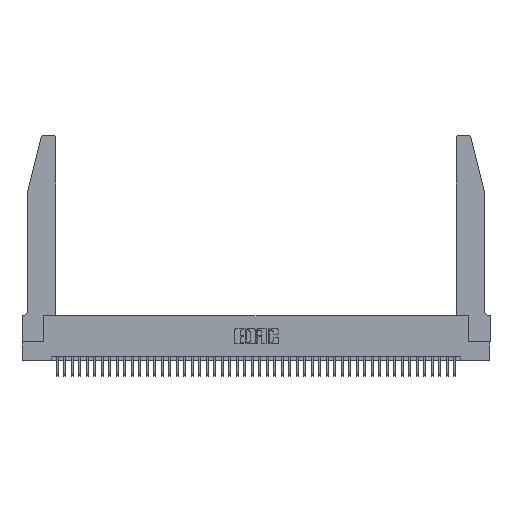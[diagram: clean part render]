
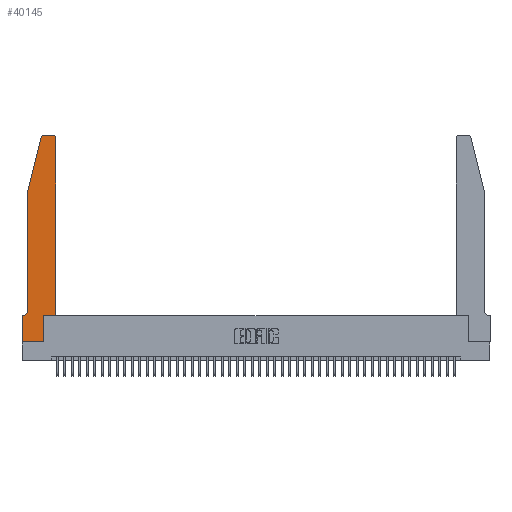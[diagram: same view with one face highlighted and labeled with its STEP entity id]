
A CAD part, top view. The second image highlights one B-rep face of the part: STEP entity #40145.
In plain terms, the highlighted planar face has unit normal (0, 0, 1).
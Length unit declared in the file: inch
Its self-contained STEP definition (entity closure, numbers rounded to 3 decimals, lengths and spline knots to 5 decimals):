
#1149 = CARTESIAN_POINT ( 'NONE',  ( 0., 0.35, 0.37 ) ) ;
#2690 = EDGE_CURVE ( 'NONE', #42190, #14684, #43488, .T. ) ;
#4485 = CIRCLE ( 'NONE', #15224, 0.03 ) ;
#4643 = EDGE_CURVE ( 'NONE', #12911, #24171, #44346, .T. ) ;
#5309 = CARTESIAN_POINT ( 'NONE',  ( 0.4505, 2.72, 0.37 ) ) ;
#5508 = ORIENTED_EDGE ( 'NONE', *, *, #18669, .T. ) ;
#6782 = CARTESIAN_POINT ( 'NONE',  ( 0., 0., 0.37 ) ) ;
#6823 = CARTESIAN_POINT ( 'NONE',  ( 0.284, 2.72, 0.37 ) ) ;
#7872 = DIRECTION ( 'NONE',  ( -0.239, -0.971, 0. ) ) ;
#8653 = DIRECTION ( 'NONE',  ( 0., 0., 1. ) ) ;
#9303 = ORIENTED_EDGE ( 'NONE', *, *, #38729, .T. ) ;
#9536 = DIRECTION ( 'NONE',  ( 0., 1., 0. ) ) ;
#9613 = CARTESIAN_POINT ( 'NONE',  ( 0.0755, 0.35, 0.37 ) ) ;
#9646 = LINE ( 'NONE', #9613, #37613 ) ;
#10460 = DIRECTION ( 'NONE',  ( 0., -1., 0. ) ) ;
#10482 = DIRECTION ( 'NONE',  ( 1., 0., 0. ) ) ;
#10718 = EDGE_CURVE ( 'NONE', #15310, #32515, #4485, .T. ) ;
#11464 = PLANE ( 'NONE',  #16009 ) ;
#11656 = VECTOR ( 'NONE', #9536, 39.37008 ) ;
#11765 = VERTEX_POINT ( 'NONE', #22542 ) ;
#12030 = DIRECTION ( 'NONE',  ( 1., 0., 0. ) ) ;
#12661 = CARTESIAN_POINT ( 'NONE',  ( 0.2865, 0., 0.37 ) ) ;
#12784 = LINE ( 'NONE', #24050, #11656 ) ;
#12911 = VERTEX_POINT ( 'NONE', #18610 ) ;
#13433 = EDGE_CURVE ( 'NONE', #22866, #42190, #46247, .T. ) ;
#13465 = ORIENTED_EDGE ( 'NONE', *, *, #39003, .T. ) ;
#13573 = CARTESIAN_POINT ( 'NONE',  ( 0.0055, 0.35, 0.37 ) ) ;
#13645 = EDGE_CURVE ( 'NONE', #11765, #12911, #18874, .T. ) ;
#13788 = DIRECTION ( 'NONE',  ( 0., 0., -1. ) ) ;
#14058 = ORIENTED_EDGE ( 'NONE', *, *, #30749, .T. ) ;
#14481 = ORIENTED_EDGE ( 'NONE', *, *, #27115, .T. ) ;
#14684 = VERTEX_POINT ( 'NONE', #12661 ) ;
#15037 = ORIENTED_EDGE ( 'NONE', *, *, #2690, .T. ) ;
#15076 = CARTESIAN_POINT ( 'NONE',  ( 0., 0.35, 0.37 ) ) ;
#15091 = EDGE_LOOP ( 'NONE', ( #13465, #14058, #28587, #16502, #9303, #5508, #37597, #15037, #14481, #41080, #19085, #21383 ) ) ;
#15224 = AXIS2_PLACEMENT_3D ( 'NONE', #30553, #8653, #34212 ) ;
#15310 = VERTEX_POINT ( 'NONE', #5309 ) ;
#16009 = AXIS2_PLACEMENT_3D ( 'NONE', #15076, #18763, #44260 ) ;
#16502 = ORIENTED_EDGE ( 'NONE', *, *, #4643, .T. ) ;
#17040 = CARTESIAN_POINT ( 'NONE',  ( 0., 0., 0.37 ) ) ;
#17180 = VECTOR ( 'NONE', #10460, 39.37008 ) ;
#18610 = CARTESIAN_POINT ( 'NONE',  ( 0.0755, 2., 0.37 ) ) ;
#18669 = EDGE_CURVE ( 'NONE', #44955, #22866, #9646, .T. ) ;
#18759 = CARTESIAN_POINT ( 'NONE',  ( 0.2865, 0.35, 0.37 ) ) ;
#18763 = DIRECTION ( 'NONE',  ( 0., 0., 1. ) ) ;
#18874 = LINE ( 'NONE', #29787, #37145 ) ;
#19085 = ORIENTED_EDGE ( 'NONE', *, *, #24826, .T. ) ;
#19884 = VERTEX_POINT ( 'NONE', #42205 ) ;
#20362 = EDGE_CURVE ( 'NONE', #42972, #24442, #25462, .T. ) ;
#20720 = DIRECTION ( 'NONE',  ( 1., 0., 0. ) ) ;
#21383 = ORIENTED_EDGE ( 'NONE', *, *, #10718, .T. ) ;
#22379 = CARTESIAN_POINT ( 'NONE',  ( 0.2605, 2.75, 0.37 ) ) ;
#22542 = CARTESIAN_POINT ( 'NONE',  ( 0.25487, 2.72718, 0.37 ) ) ;
#22866 = VERTEX_POINT ( 'NONE', #1149 ) ;
#23993 = VECTOR ( 'NONE', #44049, 39.37008 ) ;
#24050 = CARTESIAN_POINT ( 'NONE',  ( 0.4505, 0.35, 0.37 ) ) ;
#24112 = VECTOR ( 'NONE', #20720, 39.37008 ) ;
#24171 = VERTEX_POINT ( 'NONE', #26197 ) ;
#24442 = VERTEX_POINT ( 'NONE', #25032 ) ;
#24711 = CIRCLE ( 'NONE', #46565, 0.03 ) ;
#24822 = CARTESIAN_POINT ( 'NONE',  ( 0.4205, 2.75, 0.37 ) ) ;
#24826 = EDGE_CURVE ( 'NONE', #24442, #15310, #12784, .T. ) ;
#25032 = CARTESIAN_POINT ( 'NONE',  ( 0.4505, 0.35, 0.37 ) ) ;
#25462 = LINE ( 'NONE', #37558, #32904 ) ;
#25911 = CARTESIAN_POINT ( 'NONE',  ( 0.2865, 0.35, 0.37 ) ) ;
#26197 = CARTESIAN_POINT ( 'NONE',  ( 0.0755, 0.42, 0.37 ) ) ;
#26910 = CIRCLE ( 'NONE', #37708, 0.07 ) ;
#27115 = EDGE_CURVE ( 'NONE', #14684, #42972, #38783, .T. ) ;
#28587 = ORIENTED_EDGE ( 'NONE', *, *, #13645, .T. ) ;
#29787 = CARTESIAN_POINT ( 'NONE',  ( 0.0755, 2., 0.37 ) ) ;
#30553 = CARTESIAN_POINT ( 'NONE',  ( 0.4205, 2.72, 0.37 ) ) ;
#30749 = EDGE_CURVE ( 'NONE', #19884, #11765, #24711, .T. ) ;
#31511 = DIRECTION ( 'NONE',  ( -1., 0., 0. ) ) ;
#32378 = DIRECTION ( 'NONE',  ( 0., 0., 1. ) ) ;
#32515 = VERTEX_POINT ( 'NONE', #24822 ) ;
#32904 = VECTOR ( 'NONE', #12030, 39.37008 ) ;
#33124 = DIRECTION ( 'NONE',  ( 0., 1., 0. ) ) ;
#34212 = DIRECTION ( 'NONE',  ( 1., 0., 0. ) ) ;
#34709 = VECTOR ( 'NONE', #38648, 39.37008 ) ;
#35038 = CARTESIAN_POINT ( 'NONE',  ( 0.0755, 2., 0.37 ) ) ;
#35674 = CARTESIAN_POINT ( 'NONE',  ( 0.0055, 0.42, 0.37 ) ) ;
#37145 = VECTOR ( 'NONE', #7872, 39.37008 ) ;
#37558 = CARTESIAN_POINT ( 'NONE',  ( 0.4505, 0.35, 0.37 ) ) ;
#37597 = ORIENTED_EDGE ( 'NONE', *, *, #13433, .T. ) ;
#37613 = VECTOR ( 'NONE', #31511, 39.37008 ) ;
#37655 = VECTOR ( 'NONE', #33124, 39.37008 ) ;
#37708 = AXIS2_PLACEMENT_3D ( 'NONE', #35674, #13788, #39301 ) ;
#38648 = DIRECTION ( 'NONE',  ( 0., -1., 0. ) ) ;
#38729 = EDGE_CURVE ( 'NONE', #24171, #44955, #26910, .T. ) ;
#38783 = LINE ( 'NONE', #25911, #37655 ) ;
#39003 = EDGE_CURVE ( 'NONE', #32515, #19884, #43375, .T. ) ;
#39301 = DIRECTION ( 'NONE',  ( -1., 0., 0. ) ) ;
#40145 = ADVANCED_FACE ( 'NONE', ( #43824 ), #11464, .T. ) ;
#41080 = ORIENTED_EDGE ( 'NONE', *, *, #20362, .T. ) ;
#42190 = VERTEX_POINT ( 'NONE', #47021 ) ;
#42205 = CARTESIAN_POINT ( 'NONE',  ( 0.284, 2.75, 0.37 ) ) ;
#42972 = VERTEX_POINT ( 'NONE', #18759 ) ;
#43375 = LINE ( 'NONE', #22379, #23993 ) ;
#43488 = LINE ( 'NONE', #17040, #24112 ) ;
#43824 = FACE_OUTER_BOUND ( 'NONE', #15091, .T. ) ;
#44049 = DIRECTION ( 'NONE',  ( -1., 0., 0. ) ) ;
#44260 = DIRECTION ( 'NONE',  ( 1., 0., 0. ) ) ;
#44346 = LINE ( 'NONE', #35038, #34709 ) ;
#44955 = VERTEX_POINT ( 'NONE', #13573 ) ;
#46247 = LINE ( 'NONE', #6782, #17180 ) ;
#46565 = AXIS2_PLACEMENT_3D ( 'NONE', #6823, #32378, #10482 ) ;
#47021 = CARTESIAN_POINT ( 'NONE',  ( 0., 0., 0.37 ) ) ;
